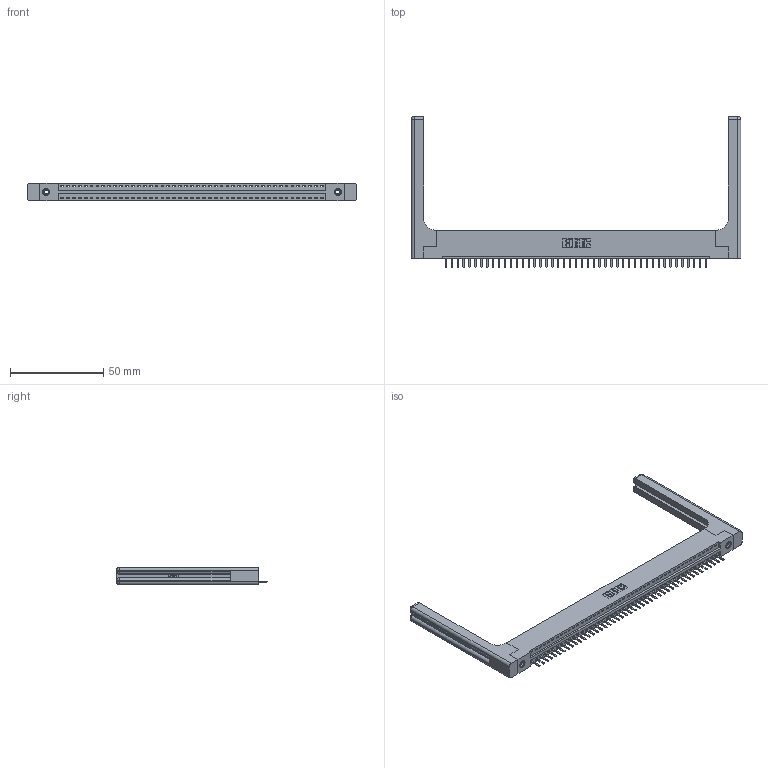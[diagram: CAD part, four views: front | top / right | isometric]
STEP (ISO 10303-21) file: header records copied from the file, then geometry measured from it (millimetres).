
FILE_DESCRIPTION (( 'STEP AP203' ), '1' );
FILE_NAME ('396-045-520-158.STEP', '2019-10-28T00:14:07', ( '' ), ( '' ), 'SwSTEP 2.0', 'SolidWorks 2016', '' );
FILE_SCHEMA (( 'CONFIG_CONTROL_DESIGN' ));
Length unit declared in the file: inch
Products named in the file (5): 345-250-001_345-250-001-102; 346 Part_Flush Mounting Lugs - 0.156 Dia-TH; 396-045-520-158; 345-292-001_345-293-120; 346-220-058_345-220-058
Assembly tree (50 placements, depth 2):
  396-045-520-158
    346 Part_Flush Mounting Lugs - 0.156 Dia-TH
    345-292-001_345-293-120  x45
    345-250-001_345-250-001-102  x2
    346-220-058_345-220-058  x2
Bounding box: 176.94 x 80.98 x 9.4 mm (x, y, z)
Volume: 24346.3 mm3; surface area: 25802.6 mm2
Topology: 50 solids, 50 shells, 3168 faces, 9275 edges, 6042 vertices
Faces by surface type: plane 2114, cylinder 994, bspline 36, cone 12, sphere 8, torus 4
Entity records: 32820 total; most frequent: CARTESIAN_POINT 6616, ORIENTED_EDGE 5380, DIRECTION 4752, EDGE_CURVE 2690, LINE 2282, VECTOR 2282, VERTEX_POINT 1782, AXIS2_PLACEMENT_3D 1235
